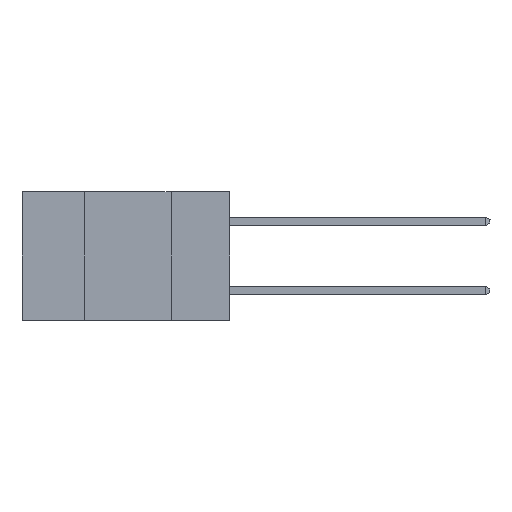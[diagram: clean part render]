
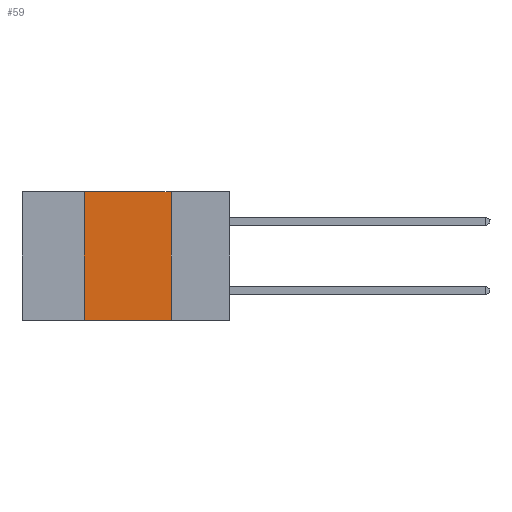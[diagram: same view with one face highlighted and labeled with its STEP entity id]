
A CAD part, left-side view. The second image highlights one B-rep face of the part: STEP entity #59.
In plain terms, the highlighted planar face has unit normal (-1, 0, 0).
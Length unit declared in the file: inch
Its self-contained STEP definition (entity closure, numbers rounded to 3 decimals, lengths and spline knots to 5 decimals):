
#59 = ADVANCED_FACE ( 'NONE', ( #5192 ), #4332, .F. ) ;
#91 = VERTEX_POINT ( 'NONE', #9664 ) ;
#419 = CARTESIAN_POINT ( 'NONE',  ( 0., 0.42, 0. ) ) ;
#778 = EDGE_CURVE ( 'NONE', #91, #10104, #8388, .T. ) ;
#1395 = LINE ( 'NONE', #419, #5433 ) ;
#1462 = VECTOR ( 'NONE', #8821, 39.37008 ) ;
#1646 = ORIENTED_EDGE ( 'NONE', *, *, #3766, .F. ) ;
#2366 = ORIENTED_EDGE ( 'NONE', *, *, #7058, .T. ) ;
#2766 = DIRECTION ( 'NONE',  ( 0., -1., 0. ) ) ;
#3164 = CARTESIAN_POINT ( 'NONE',  ( 0., 0.6, -0.37 ) ) ;
#3200 = LINE ( 'NONE', #13851, #10807 ) ;
#3766 = EDGE_CURVE ( 'NONE', #10721, #91, #1395, .T. ) ;
#4332 = PLANE ( 'NONE',  #10892 ) ;
#5192 = FACE_OUTER_BOUND ( 'NONE', #5295, .T. ) ;
#5295 = EDGE_LOOP ( 'NONE', ( #9793, #5882, #1646, #2366 ) ) ;
#5433 = VECTOR ( 'NONE', #8095, 39.37008 ) ;
#5692 = LINE ( 'NONE', #3164, #1462 ) ;
#5882 = ORIENTED_EDGE ( 'NONE', *, *, #778, .F. ) ;
#6322 = CARTESIAN_POINT ( 'NONE',  ( 0., 0.17, -0.37 ) ) ;
#7058 = EDGE_CURVE ( 'NONE', #10721, #7836, #5692, .T. ) ;
#7191 = CARTESIAN_POINT ( 'NONE',  ( 0., 0.42, -0.37 ) ) ;
#7475 = DIRECTION ( 'NONE',  ( 1., 0., 0. ) ) ;
#7836 = VERTEX_POINT ( 'NONE', #6322 ) ;
#8048 = CARTESIAN_POINT ( 'NONE',  ( 0., 0.6, 0. ) ) ;
#8095 = DIRECTION ( 'NONE',  ( 0., 0., 1. ) ) ;
#8111 = CARTESIAN_POINT ( 'NONE',  ( 0., 0.17, 0. ) ) ;
#8388 = LINE ( 'NONE', #8048, #9399 ) ;
#8821 = DIRECTION ( 'NONE',  ( 0., -1., 0. ) ) ;
#9399 = VECTOR ( 'NONE', #2766, 39.37008 ) ;
#9664 = CARTESIAN_POINT ( 'NONE',  ( 0., 0.42, 0. ) ) ;
#9793 = ORIENTED_EDGE ( 'NONE', *, *, #11126, .F. ) ;
#10104 = VERTEX_POINT ( 'NONE', #8111 ) ;
#10721 = VERTEX_POINT ( 'NONE', #7191 ) ;
#10807 = VECTOR ( 'NONE', #12698, 39.37008 ) ;
#10892 = AXIS2_PLACEMENT_3D ( 'NONE', #12999, #7475, #13924 ) ;
#11126 = EDGE_CURVE ( 'NONE', #10104, #7836, #3200, .T. ) ;
#12698 = DIRECTION ( 'NONE',  ( 0., 0., -1. ) ) ;
#12999 = CARTESIAN_POINT ( 'NONE',  ( 0., 0.6, 0. ) ) ;
#13851 = CARTESIAN_POINT ( 'NONE',  ( 0., 0.17, 0. ) ) ;
#13924 = DIRECTION ( 'NONE',  ( 0., 0., -1. ) ) ;
